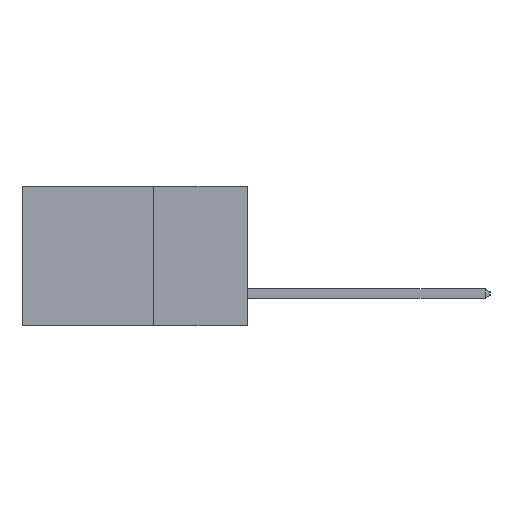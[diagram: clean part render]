
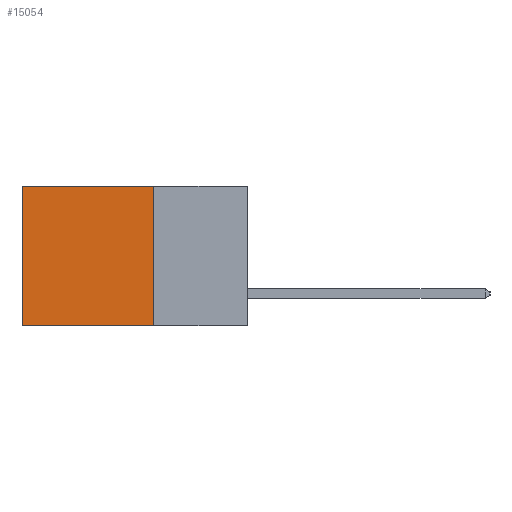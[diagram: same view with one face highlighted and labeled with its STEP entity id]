
A CAD part, left-side view. The second image highlights one B-rep face of the part: STEP entity #15054.
In plain terms, the highlighted planar face has unit normal (-1, 0, 0).
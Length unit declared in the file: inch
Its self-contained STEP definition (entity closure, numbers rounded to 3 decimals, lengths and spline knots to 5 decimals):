
#186 = ORIENTED_EDGE ( 'NONE', *, *, #15383, .T. ) ;
#194 = ORIENTED_EDGE ( 'NONE', *, *, #20197, .F. ) ;
#389 = ORIENTED_EDGE ( 'NONE', *, *, #20952, .T. ) ;
#1091 = VECTOR ( 'NONE', #13961, 39.37008 ) ;
#1484 = LINE ( 'NONE', #5353, #10113 ) ;
#2848 = DIRECTION ( 'NONE',  ( 0., 1., 0. ) ) ;
#3839 = EDGE_LOOP ( 'NONE', ( #389, #194, #13440, #186 ) ) ;
#3909 = LINE ( 'NONE', #8394, #16577 ) ;
#5353 = CARTESIAN_POINT ( 'NONE',  ( 0.2615, 0.6, -0.37 ) ) ;
#8182 = VERTEX_POINT ( 'NONE', #15659 ) ;
#8240 = DIRECTION ( 'NONE',  ( 0., 1., 0. ) ) ;
#8394 = CARTESIAN_POINT ( 'NONE',  ( 0.2615, 0.25, 0. ) ) ;
#10113 = VECTOR ( 'NONE', #10572, 39.37008 ) ;
#10572 = DIRECTION ( 'NONE',  ( 0., 0., -1. ) ) ;
#10893 = VERTEX_POINT ( 'NONE', #20662 ) ;
#12997 = AXIS2_PLACEMENT_3D ( 'NONE', #16050, #16027, #15987 ) ;
#13440 = ORIENTED_EDGE ( 'NONE', *, *, #17618, .F. ) ;
#13961 = DIRECTION ( 'NONE',  ( 0., 0., -1. ) ) ;
#14022 = CARTESIAN_POINT ( 'NONE',  ( 0.2615, 0.25, -0.37 ) ) ;
#14035 = CARTESIAN_POINT ( 'NONE',  ( 0.2615, 0.25, -0.37 ) ) ;
#14437 = FACE_OUTER_BOUND ( 'NONE', #3839, .T. ) ;
#14730 = LINE ( 'NONE', #21487, #19680 ) ;
#14850 = LINE ( 'NONE', #14035, #1091 ) ;
#15054 = ADVANCED_FACE ( 'NONE', ( #14437 ), #16380, .F. ) ;
#15383 = EDGE_CURVE ( 'NONE', #10893, #21691, #3909, .T. ) ;
#15659 = CARTESIAN_POINT ( 'NONE',  ( 0.2615, 0.6, -0.37 ) ) ;
#15987 = DIRECTION ( 'NONE',  ( 0., 0., -1. ) ) ;
#16027 = DIRECTION ( 'NONE',  ( 1., 0., 0. ) ) ;
#16050 = CARTESIAN_POINT ( 'NONE',  ( 0.2615, 0.25, -0.37 ) ) ;
#16380 = PLANE ( 'NONE',  #12997 ) ;
#16577 = VECTOR ( 'NONE', #8240, 39.37008 ) ;
#17618 = EDGE_CURVE ( 'NONE', #10893, #20959, #14850, .T. ) ;
#18634 = CARTESIAN_POINT ( 'NONE',  ( 0.2615, 0.6, 0. ) ) ;
#19680 = VECTOR ( 'NONE', #2848, 39.37008 ) ;
#20197 = EDGE_CURVE ( 'NONE', #20959, #8182, #14730, .T. ) ;
#20662 = CARTESIAN_POINT ( 'NONE',  ( 0.2615, 0.25, 0. ) ) ;
#20952 = EDGE_CURVE ( 'NONE', #21691, #8182, #1484, .T. ) ;
#20959 = VERTEX_POINT ( 'NONE', #14022 ) ;
#21487 = CARTESIAN_POINT ( 'NONE',  ( 0.2615, 0.25, -0.37 ) ) ;
#21691 = VERTEX_POINT ( 'NONE', #18634 ) ;
